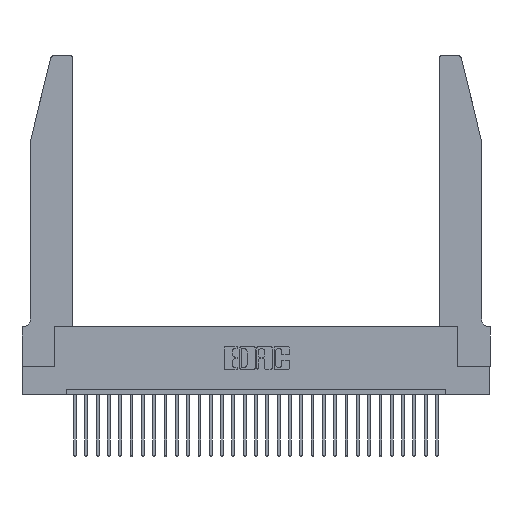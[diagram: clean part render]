
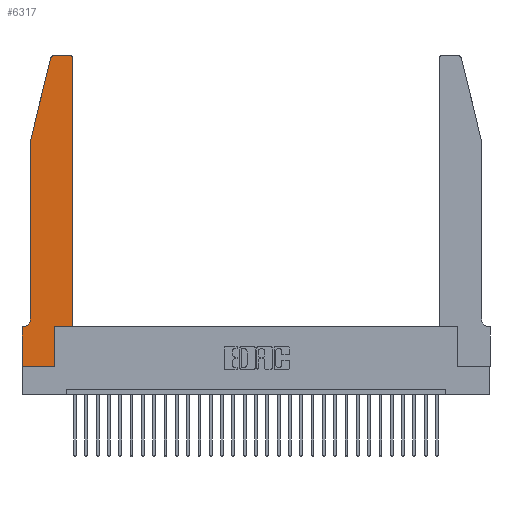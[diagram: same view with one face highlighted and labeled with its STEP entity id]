
A CAD part, top view. The second image highlights one B-rep face of the part: STEP entity #6317.
In plain terms, the highlighted planar face has unit normal (0, 0, 1).
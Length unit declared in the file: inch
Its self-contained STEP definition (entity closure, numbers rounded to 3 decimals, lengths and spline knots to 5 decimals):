
#11 = VECTOR ( 'NONE', #20260, 39.37008 ) ;
#53 = DIRECTION ( 'NONE',  ( 1., 0., 0. ) ) ;
#70 = FACE_OUTER_BOUND ( 'NONE', #11833, .T. ) ;
#365 = VERTEX_POINT ( 'NONE', #24761 ) ;
#452 = ORIENTED_EDGE ( 'NONE', *, *, #27794, .T. ) ;
#635 = VERTEX_POINT ( 'NONE', #21403 ) ;
#909 = DIRECTION ( 'NONE',  ( -1., 0., 0. ) ) ;
#1429 = CARTESIAN_POINT ( 'NONE',  ( 0.25487, 2.72718, 0.37 ) ) ;
#1539 = ORIENTED_EDGE ( 'NONE', *, *, #17830, .T. ) ;
#1733 = VERTEX_POINT ( 'NONE', #16702 ) ;
#2719 = VERTEX_POINT ( 'NONE', #21507 ) ;
#3065 = VERTEX_POINT ( 'NONE', #13153 ) ;
#3400 = VERTEX_POINT ( 'NONE', #25930 ) ;
#3413 = AXIS2_PLACEMENT_3D ( 'NONE', #4024, #13564, #29144 ) ;
#3625 = LINE ( 'NONE', #22669, #12186 ) ;
#3631 = CARTESIAN_POINT ( 'NONE',  ( 0.0755, 2., 0.37 ) ) ;
#3772 = EDGE_CURVE ( 'NONE', #10564, #3065, #10642, .T. ) ;
#4024 = CARTESIAN_POINT ( 'NONE',  ( 0., 0.35, 0.37 ) ) ;
#4531 = ORIENTED_EDGE ( 'NONE', *, *, #26679, .T. ) ;
#4700 = ORIENTED_EDGE ( 'NONE', *, *, #10550, .T. ) ;
#4999 = CARTESIAN_POINT ( 'NONE',  ( 0.2865, 0.35, 0.37 ) ) ;
#5749 = CIRCLE ( 'NONE', #10837, 0.03 ) ;
#6317 = ADVANCED_FACE ( 'NONE', ( #70 ), #9686, .T. ) ;
#7247 = ORIENTED_EDGE ( 'NONE', *, *, #8827, .T. ) ;
#7632 = VECTOR ( 'NONE', #15776, 39.37008 ) ;
#7890 = LINE ( 'NONE', #14195, #18683 ) ;
#8222 = CARTESIAN_POINT ( 'NONE',  ( 0.4505, 2.72, 0.37 ) ) ;
#8262 = EDGE_CURVE ( 'NONE', #26072, #365, #8543, .T. ) ;
#8543 = LINE ( 'NONE', #28161, #23411 ) ;
#8827 = EDGE_CURVE ( 'NONE', #1733, #12562, #11099, .T. ) ;
#9444 = LINE ( 'NONE', #4999, #27681 ) ;
#9566 = VECTOR ( 'NONE', #27141, 39.37008 ) ;
#9569 = CARTESIAN_POINT ( 'NONE',  ( 0.284, 2.72, 0.37 ) ) ;
#9686 = PLANE ( 'NONE',  #3413 ) ;
#10363 = VECTOR ( 'NONE', #14621, 39.37008 ) ;
#10550 = EDGE_CURVE ( 'NONE', #15454, #635, #24420, .T. ) ;
#10564 = VERTEX_POINT ( 'NONE', #8222 ) ;
#10642 = CIRCLE ( 'NONE', #27452, 0.03 ) ;
#10754 = CARTESIAN_POINT ( 'NONE',  ( 0.2865, 0., 0.37 ) ) ;
#10837 = AXIS2_PLACEMENT_3D ( 'NONE', #9569, #16816, #53 ) ;
#11099 = LINE ( 'NONE', #14130, #10363 ) ;
#11609 = DIRECTION ( 'NONE',  ( -1., 0., 0. ) ) ;
#11833 = EDGE_LOOP ( 'NONE', ( #4531, #30814, #4700, #452, #1539, #24653, #7247, #30197, #21431, #26925, #15261, #27070 ) ) ;
#12078 = CARTESIAN_POINT ( 'NONE',  ( 0.2865, 0.35, 0.37 ) ) ;
#12186 = VECTOR ( 'NONE', #12924, 39.37008 ) ;
#12562 = VERTEX_POINT ( 'NONE', #24633 ) ;
#12877 = EDGE_CURVE ( 'NONE', #365, #10564, #27327, .T. ) ;
#12924 = DIRECTION ( 'NONE',  ( -1., 0., 0. ) ) ;
#12989 = CARTESIAN_POINT ( 'NONE',  ( 0.0055, 0.42, 0.37 ) ) ;
#13153 = CARTESIAN_POINT ( 'NONE',  ( 0.4205, 2.75, 0.37 ) ) ;
#13564 = DIRECTION ( 'NONE',  ( 0., 0., 1. ) ) ;
#13948 = LINE ( 'NONE', #15351, #7632 ) ;
#13992 = VERTEX_POINT ( 'NONE', #10754 ) ;
#14130 = CARTESIAN_POINT ( 'NONE',  ( 0., 0., 0.37 ) ) ;
#14195 = CARTESIAN_POINT ( 'NONE',  ( 0.2605, 2.75, 0.37 ) ) ;
#14621 = DIRECTION ( 'NONE',  ( 0., -1., 0. ) ) ;
#14647 = VECTOR ( 'NONE', #24973, 39.37008 ) ;
#15261 = ORIENTED_EDGE ( 'NONE', *, *, #12877, .T. ) ;
#15351 = CARTESIAN_POINT ( 'NONE',  ( 0., 0., 0.37 ) ) ;
#15454 = VERTEX_POINT ( 'NONE', #1429 ) ;
#15776 = DIRECTION ( 'NONE',  ( 1., 0., 0. ) ) ;
#16412 = DIRECTION ( 'NONE',  ( 0., 0., 1. ) ) ;
#16702 = CARTESIAN_POINT ( 'NONE',  ( 0., 0.35, 0.37 ) ) ;
#16816 = DIRECTION ( 'NONE',  ( 0., 0., 1. ) ) ;
#17649 = CARTESIAN_POINT ( 'NONE',  ( 0.0755, 2., 0.37 ) ) ;
#17830 = EDGE_CURVE ( 'NONE', #20919, #3400, #27108, .T. ) ;
#18108 = CARTESIAN_POINT ( 'NONE',  ( 0.0755, 0.42, 0.37 ) ) ;
#18683 = VECTOR ( 'NONE', #11609, 39.37008 ) ;
#18970 = DIRECTION ( 'NONE',  ( 0., 1., 0. ) ) ;
#19035 = EDGE_CURVE ( 'NONE', #3400, #1733, #3625, .T. ) ;
#19537 = AXIS2_PLACEMENT_3D ( 'NONE', #12989, #22632, #909 ) ;
#20260 = DIRECTION ( 'NONE',  ( 0., -1., 0. ) ) ;
#20553 = EDGE_CURVE ( 'NONE', #12562, #13992, #13948, .T. ) ;
#20769 = EDGE_CURVE ( 'NONE', #2719, #15454, #5749, .T. ) ;
#20919 = VERTEX_POINT ( 'NONE', #18108 ) ;
#21403 = CARTESIAN_POINT ( 'NONE',  ( 0.0755, 2., 0.37 ) ) ;
#21431 = ORIENTED_EDGE ( 'NONE', *, *, #26027, .T. ) ;
#21507 = CARTESIAN_POINT ( 'NONE',  ( 0.284, 2.75, 0.37 ) ) ;
#22632 = DIRECTION ( 'NONE',  ( 0., 0., -1. ) ) ;
#22669 = CARTESIAN_POINT ( 'NONE',  ( 0.0755, 0.35, 0.37 ) ) ;
#23411 = VECTOR ( 'NONE', #30621, 39.37008 ) ;
#24420 = LINE ( 'NONE', #17649, #9566 ) ;
#24580 = LINE ( 'NONE', #3631, #11 ) ;
#24633 = CARTESIAN_POINT ( 'NONE',  ( 0., 0., 0.37 ) ) ;
#24653 = ORIENTED_EDGE ( 'NONE', *, *, #19035, .T. ) ;
#24761 = CARTESIAN_POINT ( 'NONE',  ( 0.4505, 0.35, 0.37 ) ) ;
#24973 = DIRECTION ( 'NONE',  ( 0., 1., 0. ) ) ;
#25275 = CARTESIAN_POINT ( 'NONE',  ( 0.4505, 0.35, 0.37 ) ) ;
#25930 = CARTESIAN_POINT ( 'NONE',  ( 0.0055, 0.35, 0.37 ) ) ;
#26027 = EDGE_CURVE ( 'NONE', #13992, #26072, #9444, .T. ) ;
#26072 = VERTEX_POINT ( 'NONE', #12078 ) ;
#26679 = EDGE_CURVE ( 'NONE', #3065, #2719, #7890, .T. ) ;
#26925 = ORIENTED_EDGE ( 'NONE', *, *, #8262, .T. ) ;
#27070 = ORIENTED_EDGE ( 'NONE', *, *, #3772, .T. ) ;
#27108 = CIRCLE ( 'NONE', #19537, 0.07 ) ;
#27141 = DIRECTION ( 'NONE',  ( -0.239, -0.971, 0. ) ) ;
#27327 = LINE ( 'NONE', #25275, #14647 ) ;
#27452 = AXIS2_PLACEMENT_3D ( 'NONE', #28665, #16412, #30736 ) ;
#27681 = VECTOR ( 'NONE', #18970, 39.37008 ) ;
#27794 = EDGE_CURVE ( 'NONE', #635, #20919, #24580, .T. ) ;
#28161 = CARTESIAN_POINT ( 'NONE',  ( 0.4505, 0.35, 0.37 ) ) ;
#28665 = CARTESIAN_POINT ( 'NONE',  ( 0.4205, 2.72, 0.37 ) ) ;
#29144 = DIRECTION ( 'NONE',  ( 1., 0., 0. ) ) ;
#30197 = ORIENTED_EDGE ( 'NONE', *, *, #20553, .T. ) ;
#30621 = DIRECTION ( 'NONE',  ( 1., 0., 0. ) ) ;
#30736 = DIRECTION ( 'NONE',  ( 1., 0., 0. ) ) ;
#30814 = ORIENTED_EDGE ( 'NONE', *, *, #20769, .T. ) ;
